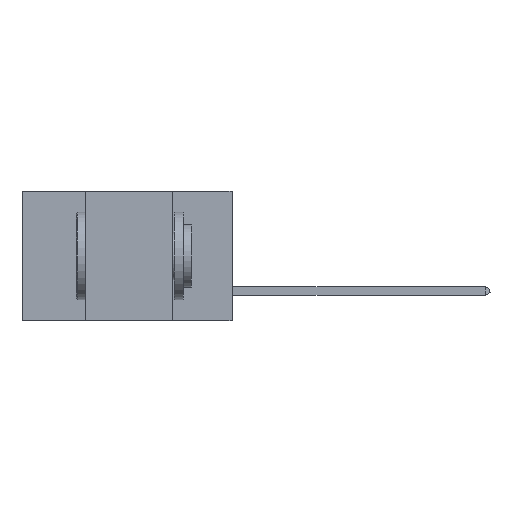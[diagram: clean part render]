
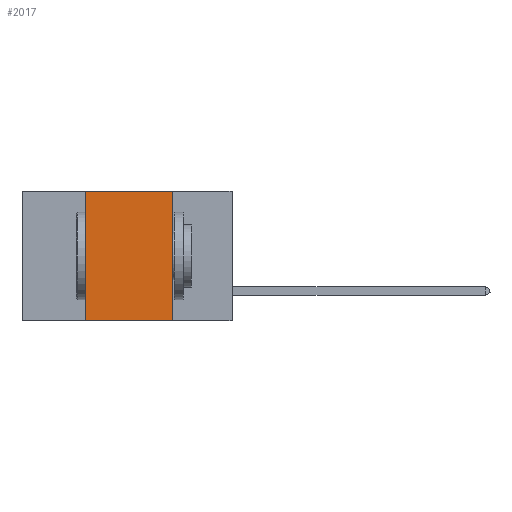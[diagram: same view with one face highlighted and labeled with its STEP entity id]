
A CAD part, left-side view. The second image highlights one B-rep face of the part: STEP entity #2017.
In plain terms, the highlighted planar face has unit normal (-1, 0, 0).
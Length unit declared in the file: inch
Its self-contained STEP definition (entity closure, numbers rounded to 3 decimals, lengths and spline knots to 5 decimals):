
#405 = LINE ( 'NONE', #8553, #2063 ) ;
#502 = ORIENTED_EDGE ( 'NONE', *, *, #1670, .F. ) ;
#615 = ORIENTED_EDGE ( 'NONE', *, *, #2948, .F. ) ;
#1066 = CARTESIAN_POINT ( 'NONE',  ( 0., 0.42, 0. ) ) ;
#1086 = DIRECTION ( 'NONE',  ( 0., -1., 0. ) ) ;
#1670 = EDGE_CURVE ( 'NONE', #2908, #4848, #405, .T. ) ;
#1692 = DIRECTION ( 'NONE',  ( 0., 0., -1. ) ) ;
#2017 = ADVANCED_FACE ( 'NONE', ( #10535 ), #9966, .F. ) ;
#2043 = LINE ( 'NONE', #2171, #10125 ) ;
#2063 = VECTOR ( 'NONE', #1086, 39.37008 ) ;
#2171 = CARTESIAN_POINT ( 'NONE',  ( 0., 0.6, -0.37 ) ) ;
#2212 = DIRECTION ( 'NONE',  ( 0., -1., 0. ) ) ;
#2299 = CARTESIAN_POINT ( 'NONE',  ( 0., 0.42, 0. ) ) ;
#2873 = LINE ( 'NONE', #2299, #7561 ) ;
#2908 = VERTEX_POINT ( 'NONE', #1066 ) ;
#2948 = EDGE_CURVE ( 'NONE', #4848, #4344, #4662, .T. ) ;
#3209 = EDGE_CURVE ( 'NONE', #3890, #4344, #2043, .T. ) ;
#3427 = AXIS2_PLACEMENT_3D ( 'NONE', #6606, #7546, #1692 ) ;
#3448 = CARTESIAN_POINT ( 'NONE',  ( 0., 0.42, -0.37 ) ) ;
#3890 = VERTEX_POINT ( 'NONE', #3448 ) ;
#4344 = VERTEX_POINT ( 'NONE', #6985 ) ;
#4549 = CARTESIAN_POINT ( 'NONE',  ( 0., 0.17, 0. ) ) ;
#4662 = LINE ( 'NONE', #4549, #10131 ) ;
#4848 = VERTEX_POINT ( 'NONE', #7325 ) ;
#5436 = EDGE_LOOP ( 'NONE', ( #615, #502, #7300, #10003 ) ) ;
#5790 = DIRECTION ( 'NONE',  ( 0., 0., 1. ) ) ;
#6606 = CARTESIAN_POINT ( 'NONE',  ( 0., 0.6, 0. ) ) ;
#6985 = CARTESIAN_POINT ( 'NONE',  ( 0., 0.17, -0.37 ) ) ;
#6988 = EDGE_CURVE ( 'NONE', #3890, #2908, #2873, .T. ) ;
#6992 = DIRECTION ( 'NONE',  ( 0., 0., -1. ) ) ;
#7300 = ORIENTED_EDGE ( 'NONE', *, *, #6988, .F. ) ;
#7325 = CARTESIAN_POINT ( 'NONE',  ( 0., 0.17, 0. ) ) ;
#7546 = DIRECTION ( 'NONE',  ( 1., 0., 0. ) ) ;
#7561 = VECTOR ( 'NONE', #5790, 39.37008 ) ;
#8553 = CARTESIAN_POINT ( 'NONE',  ( 0., 0.6, 0. ) ) ;
#9966 = PLANE ( 'NONE',  #3427 ) ;
#10003 = ORIENTED_EDGE ( 'NONE', *, *, #3209, .T. ) ;
#10125 = VECTOR ( 'NONE', #2212, 39.37008 ) ;
#10131 = VECTOR ( 'NONE', #6992, 39.37008 ) ;
#10535 = FACE_OUTER_BOUND ( 'NONE', #5436, .T. ) ;
